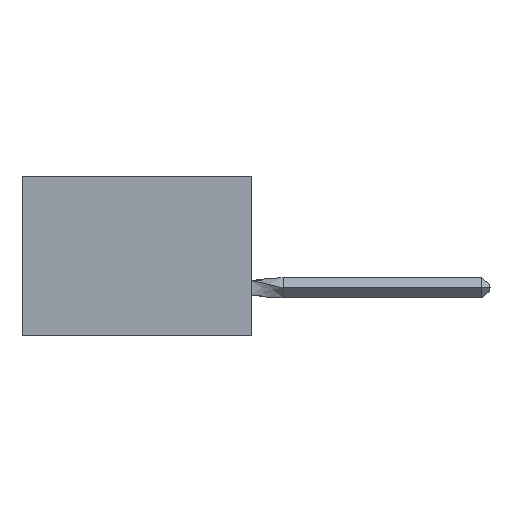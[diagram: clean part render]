
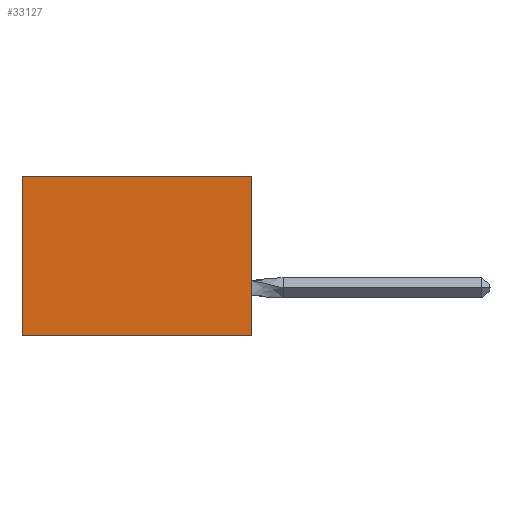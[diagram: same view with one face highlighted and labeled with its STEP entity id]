
A CAD part, left-side view. The second image highlights one B-rep face of the part: STEP entity #33127.
In plain terms, the highlighted planar face has unit normal (-1, 0, 0).
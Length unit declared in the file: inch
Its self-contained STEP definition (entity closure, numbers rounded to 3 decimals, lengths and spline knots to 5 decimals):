
#276 = CARTESIAN_POINT ( 'NONE',  ( 0.305, 0.72, -0.5 ) ) ;
#2948 = DIRECTION ( 'NONE',  ( 0., 1., 0. ) ) ;
#5195 = CARTESIAN_POINT ( 'NONE',  ( 0.305, 0.72, -0.5 ) ) ;
#6456 = PLANE ( 'NONE',  #16557 ) ;
#7344 = LINE ( 'NONE', #25383, #8325 ) ;
#8325 = VECTOR ( 'NONE', #22455, 39.37008 ) ;
#9094 = EDGE_CURVE ( 'NONE', #20755, #20226, #23115, .T. ) ;
#10622 = LINE ( 'NONE', #20233, #17584 ) ;
#10661 = EDGE_CURVE ( 'NONE', #40233, #20226, #10622, .T. ) ;
#12617 = VECTOR ( 'NONE', #2948, 39.37008 ) ;
#13176 = FACE_OUTER_BOUND ( 'NONE', #31659, .T. ) ;
#13633 = VECTOR ( 'NONE', #14392, 39.37008 ) ;
#14060 = VERTEX_POINT ( 'NONE', #17871 ) ;
#14392 = DIRECTION ( 'NONE',  ( 0., 0., -1. ) ) ;
#16397 = ORIENTED_EDGE ( 'NONE', *, *, #17011, .F. ) ;
#16557 = AXIS2_PLACEMENT_3D ( 'NONE', #21583, #40740, #22623 ) ;
#17011 = EDGE_CURVE ( 'NONE', #14060, #40233, #7344, .T. ) ;
#17584 = VECTOR ( 'NONE', #23700, 39.37008 ) ;
#17871 = CARTESIAN_POINT ( 'NONE',  ( 0.305, 0., 0. ) ) ;
#20226 = VERTEX_POINT ( 'NONE', #276 ) ;
#20233 = CARTESIAN_POINT ( 'NONE',  ( 0.305, 0., -0.5 ) ) ;
#20755 = VERTEX_POINT ( 'NONE', #24015 ) ;
#21583 = CARTESIAN_POINT ( 'NONE',  ( 0.305, 0., -0.5 ) ) ;
#22455 = DIRECTION ( 'NONE',  ( 0., 0., -1. ) ) ;
#22623 = DIRECTION ( 'NONE',  ( 0., 0., -1. ) ) ;
#23115 = LINE ( 'NONE', #5195, #13633 ) ;
#23700 = DIRECTION ( 'NONE',  ( 0., 1., 0. ) ) ;
#23833 = EDGE_CURVE ( 'NONE', #14060, #20755, #35070, .T. ) ;
#24015 = CARTESIAN_POINT ( 'NONE',  ( 0.305, 0.72, 0. ) ) ;
#24044 = ORIENTED_EDGE ( 'NONE', *, *, #23833, .T. ) ;
#25383 = CARTESIAN_POINT ( 'NONE',  ( 0.305, 0., -0.5 ) ) ;
#31659 = EDGE_LOOP ( 'NONE', ( #40438, #40497, #16397, #24044 ) ) ;
#33127 = ADVANCED_FACE ( 'NONE', ( #13176 ), #6456, .F. ) ;
#35070 = LINE ( 'NONE', #38067, #12617 ) ;
#35812 = CARTESIAN_POINT ( 'NONE',  ( 0.305, 0., -0.5 ) ) ;
#38067 = CARTESIAN_POINT ( 'NONE',  ( 0.305, 0., 0. ) ) ;
#40233 = VERTEX_POINT ( 'NONE', #35812 ) ;
#40438 = ORIENTED_EDGE ( 'NONE', *, *, #9094, .T. ) ;
#40497 = ORIENTED_EDGE ( 'NONE', *, *, #10661, .F. ) ;
#40740 = DIRECTION ( 'NONE',  ( 1., 0., 0. ) ) ;
